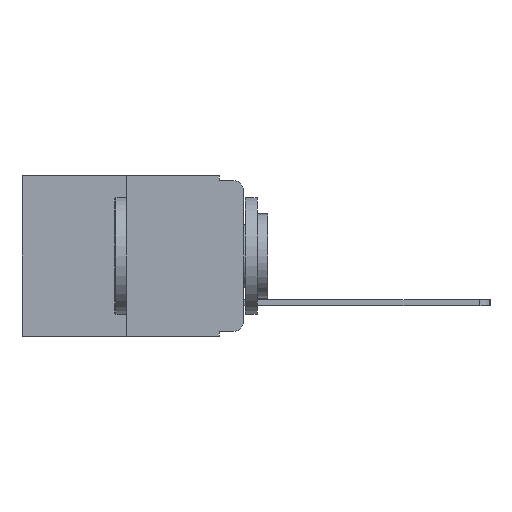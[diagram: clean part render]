
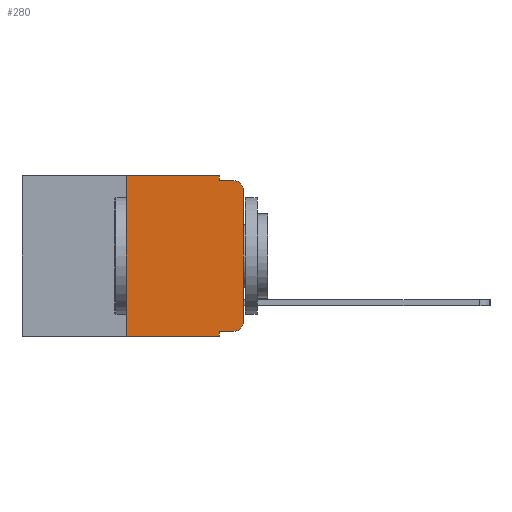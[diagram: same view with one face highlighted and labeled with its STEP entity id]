
A CAD part, left-side view. The second image highlights one B-rep face of the part: STEP entity #280.
In plain terms, the highlighted planar face has unit normal (-1, 0, 0).
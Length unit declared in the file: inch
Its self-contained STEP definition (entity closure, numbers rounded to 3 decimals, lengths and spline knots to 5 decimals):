
#40 = DIRECTION ( 'NONE',  ( 1., 0., 0. ) ) ;
#138 = ORIENTED_EDGE ( 'NONE', *, *, #8266, .F. ) ;
#160 = DIRECTION ( 'NONE',  ( 0., -1., 0. ) ) ;
#280 = ADVANCED_FACE ( 'NONE', ( #8817 ), #6972, .F. ) ;
#891 = DIRECTION ( 'NONE',  ( 0., -1., 0. ) ) ;
#964 = LINE ( 'NONE', #6663, #6085 ) ;
#1016 = EDGE_CURVE ( 'NONE', #5528, #4430, #5865, .T. ) ;
#1117 = DIRECTION ( 'NONE',  ( 0., 0., -1. ) ) ;
#1150 = LINE ( 'NONE', #11294, #5949 ) ;
#1261 = CARTESIAN_POINT ( 'NONE',  ( 0., 0.051, -0.333 ) ) ;
#1421 = ORIENTED_EDGE ( 'NONE', *, *, #9516, .F. ) ;
#1646 = DIRECTION ( 'NONE',  ( 0., -1., 0. ) ) ;
#1721 = VECTOR ( 'NONE', #12631, 39.37008 ) ;
#1951 = VERTEX_POINT ( 'NONE', #4514 ) ;
#2055 = EDGE_CURVE ( 'NONE', #5920, #10136, #9781, .T. ) ;
#2192 = DIRECTION ( 'NONE',  ( -1., 0., 0. ) ) ;
#2299 = ORIENTED_EDGE ( 'NONE', *, *, #6416, .F. ) ;
#2338 = ORIENTED_EDGE ( 'NONE', *, *, #1016, .T. ) ;
#2518 = VERTEX_POINT ( 'NONE', #3987 ) ;
#2528 = ORIENTED_EDGE ( 'NONE', *, *, #9010, .F. ) ;
#2886 = AXIS2_PLACEMENT_3D ( 'NONE', #5602, #12182, #6590 ) ;
#3228 = ORIENTED_EDGE ( 'NONE', *, *, #10769, .T. ) ;
#3314 = VERTEX_POINT ( 'NONE', #1261 ) ;
#3597 = VECTOR ( 'NONE', #160, 39.37008 ) ;
#3752 = ORIENTED_EDGE ( 'NONE', *, *, #2055, .T. ) ;
#3838 = AXIS2_PLACEMENT_3D ( 'NONE', #8130, #2192, #9067 ) ;
#3918 = LINE ( 'NONE', #11903, #3597 ) ;
#3987 = CARTESIAN_POINT ( 'NONE',  ( 0., 0.02, -0.01 ) ) ;
#4044 = ORIENTED_EDGE ( 'NONE', *, *, #5314, .F. ) ;
#4047 = CARTESIAN_POINT ( 'NONE',  ( 0., 0.25, 0. ) ) ;
#4339 = VECTOR ( 'NONE', #8735, 39.37008 ) ;
#4430 = VERTEX_POINT ( 'NONE', #8129 ) ;
#4435 = LINE ( 'NONE', #4047, #1721 ) ;
#4514 = CARTESIAN_POINT ( 'NONE',  ( 0., 0.25, 0. ) ) ;
#4631 = EDGE_LOOP ( 'NONE', ( #3752, #3228, #1421, #138, #2528, #2299, #2338, #4044, #10993, #5976 ) ) ;
#5314 = EDGE_CURVE ( 'NONE', #3314, #4430, #9999, .T. ) ;
#5316 = CARTESIAN_POINT ( 'NONE',  ( 0., 0., -0.313 ) ) ;
#5335 = DIRECTION ( 'NONE',  ( 0., 0., -1. ) ) ;
#5528 = VERTEX_POINT ( 'NONE', #9419 ) ;
#5602 = CARTESIAN_POINT ( 'NONE',  ( 0., 0.02, -0.03 ) ) ;
#5746 = DIRECTION ( 'NONE',  ( 0., 0., 1. ) ) ;
#5865 = LINE ( 'NONE', #8933, #8065 ) ;
#5920 = VERTEX_POINT ( 'NONE', #5316 ) ;
#5949 = VECTOR ( 'NONE', #9398, 39.37008 ) ;
#5976 = ORIENTED_EDGE ( 'NONE', *, *, #10612, .T. ) ;
#6085 = VECTOR ( 'NONE', #1646, 39.37008 ) ;
#6370 = CIRCLE ( 'NONE', #2886, 0.02 ) ;
#6416 = EDGE_CURVE ( 'NONE', #5528, #1951, #4435, .T. ) ;
#6590 = DIRECTION ( 'NONE',  ( 0., 0., -1. ) ) ;
#6663 = CARTESIAN_POINT ( 'NONE',  ( 0., 0.051, -0.01 ) ) ;
#6751 = VECTOR ( 'NONE', #5746, 39.37008 ) ;
#6972 = PLANE ( 'NONE',  #8321 ) ;
#6984 = LINE ( 'NONE', #12464, #4339 ) ;
#7498 = VERTEX_POINT ( 'NONE', #11978 ) ;
#8065 = VECTOR ( 'NONE', #891, 39.37008 ) ;
#8129 = CARTESIAN_POINT ( 'NONE',  ( 0., 0.051, -0.343 ) ) ;
#8130 = CARTESIAN_POINT ( 'NONE',  ( 0., 0.02, -0.313 ) ) ;
#8157 = CARTESIAN_POINT ( 'NONE',  ( 0., 0.473, 0. ) ) ;
#8266 = EDGE_CURVE ( 'NONE', #7498, #10069, #1150, .T. ) ;
#8321 = AXIS2_PLACEMENT_3D ( 'NONE', #8157, #40, #1117 ) ;
#8735 = DIRECTION ( 'NONE',  ( 0., -1., 0. ) ) ;
#8817 = FACE_OUTER_BOUND ( 'NONE', #4631, .T. ) ;
#8933 = CARTESIAN_POINT ( 'NONE',  ( 0., 0.473, -0.343 ) ) ;
#8948 = CARTESIAN_POINT ( 'NONE',  ( 0., 0.051, -0.01 ) ) ;
#9010 = EDGE_CURVE ( 'NONE', #1951, #7498, #6984, .T. ) ;
#9067 = DIRECTION ( 'NONE',  ( 0., 0., -1. ) ) ;
#9398 = DIRECTION ( 'NONE',  ( 0., 0., -1. ) ) ;
#9418 = VECTOR ( 'NONE', #5335, 39.37008 ) ;
#9419 = CARTESIAN_POINT ( 'NONE',  ( 0., 0.25, -0.343 ) ) ;
#9516 = EDGE_CURVE ( 'NONE', #10069, #2518, #964, .T. ) ;
#9553 = VERTEX_POINT ( 'NONE', #12370 ) ;
#9746 = CARTESIAN_POINT ( 'NONE',  ( 0., 0., 0. ) ) ;
#9781 = LINE ( 'NONE', #9746, #6751 ) ;
#9999 = LINE ( 'NONE', #11947, #9418 ) ;
#10069 = VERTEX_POINT ( 'NONE', #8948 ) ;
#10136 = VERTEX_POINT ( 'NONE', #10916 ) ;
#10282 = CIRCLE ( 'NONE', #3838, 0.02 ) ;
#10612 = EDGE_CURVE ( 'NONE', #9553, #5920, #10282, .T. ) ;
#10769 = EDGE_CURVE ( 'NONE', #10136, #2518, #6370, .T. ) ;
#10916 = CARTESIAN_POINT ( 'NONE',  ( 0., 0., -0.03 ) ) ;
#10993 = ORIENTED_EDGE ( 'NONE', *, *, #12504, .T. ) ;
#11294 = CARTESIAN_POINT ( 'NONE',  ( 0., 0.051, 0. ) ) ;
#11903 = CARTESIAN_POINT ( 'NONE',  ( 0., 0.051, -0.333 ) ) ;
#11947 = CARTESIAN_POINT ( 'NONE',  ( 0., 0.051, 0. ) ) ;
#11978 = CARTESIAN_POINT ( 'NONE',  ( 0., 0.051, 0. ) ) ;
#12182 = DIRECTION ( 'NONE',  ( -1., 0., 0. ) ) ;
#12370 = CARTESIAN_POINT ( 'NONE',  ( 0., 0.02, -0.333 ) ) ;
#12464 = CARTESIAN_POINT ( 'NONE',  ( 0., 0.473, 0. ) ) ;
#12504 = EDGE_CURVE ( 'NONE', #3314, #9553, #3918, .T. ) ;
#12631 = DIRECTION ( 'NONE',  ( 0., 0., 1. ) ) ;
